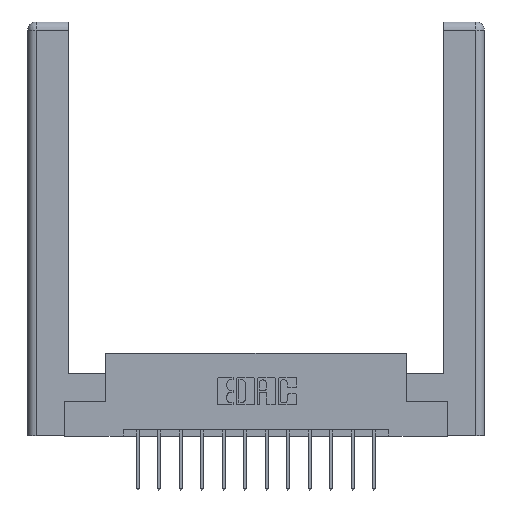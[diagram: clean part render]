
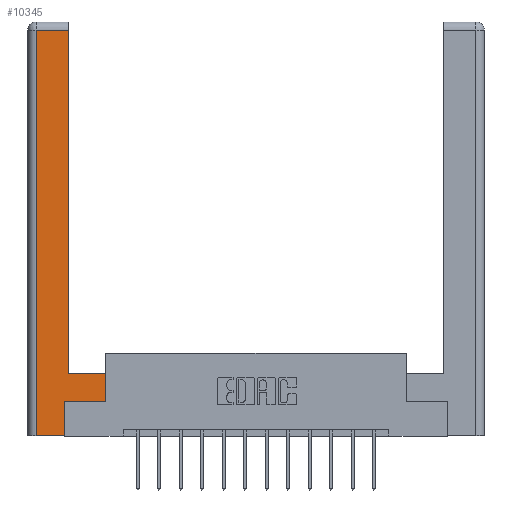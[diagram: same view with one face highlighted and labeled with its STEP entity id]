
A CAD part, top view. The second image highlights one B-rep face of the part: STEP entity #10345.
In plain terms, the highlighted planar face has unit normal (0, 0, 1).
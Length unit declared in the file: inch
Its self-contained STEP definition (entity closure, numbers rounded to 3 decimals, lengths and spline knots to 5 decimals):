
#161 = ORIENTED_EDGE ( 'NONE', *, *, #13510, .T. ) ;
#336 = DIRECTION ( 'NONE',  ( -1., 0., 0. ) ) ;
#454 = EDGE_CURVE ( 'NONE', #11372, #15323, #6470, .T. ) ;
#505 = CARTESIAN_POINT ( 'NONE',  ( 0.265, 0., 0. ) ) ;
#992 = CARTESIAN_POINT ( 'NONE',  ( 0.265, 0.245, 0. ) ) ;
#1476 = VERTEX_POINT ( 'NONE', #2406 ) ;
#1757 = VERTEX_POINT ( 'NONE', #505 ) ;
#1783 = LINE ( 'NONE', #3358, #5050 ) ;
#1943 = ORIENTED_EDGE ( 'NONE', *, *, #4255, .T. ) ;
#2093 = VECTOR ( 'NONE', #6991, 39.37008 ) ;
#2279 = VECTOR ( 'NONE', #3159, 39.37008 ) ;
#2306 = LINE ( 'NONE', #6156, #5923 ) ;
#2406 = CARTESIAN_POINT ( 'NONE',  ( 0.295, 0.45, 0. ) ) ;
#2756 = VERTEX_POINT ( 'NONE', #992 ) ;
#3066 = ORIENTED_EDGE ( 'NONE', *, *, #4370, .T. ) ;
#3159 = DIRECTION ( 'NONE',  ( 0., 1., 0. ) ) ;
#3294 = CARTESIAN_POINT ( 'NONE',  ( 0.565, 0.245, 0. ) ) ;
#3358 = CARTESIAN_POINT ( 'NONE',  ( 0.265, 0.245, 0. ) ) ;
#3514 = AXIS2_PLACEMENT_3D ( 'NONE', #7542, #14059, #6756 ) ;
#4255 = EDGE_CURVE ( 'NONE', #1476, #11372, #9552, .T. ) ;
#4336 = VERTEX_POINT ( 'NONE', #8377 ) ;
#4370 = EDGE_CURVE ( 'NONE', #15323, #4336, #6119, .T. ) ;
#4674 = DIRECTION ( 'NONE',  ( -1., 0., 0. ) ) ;
#5003 = VERTEX_POINT ( 'NONE', #10458 ) ;
#5050 = VECTOR ( 'NONE', #13098, 39.37008 ) ;
#5762 = FACE_OUTER_BOUND ( 'NONE', #10119, .T. ) ;
#5923 = VECTOR ( 'NONE', #14624, 39.37008 ) ;
#6119 = LINE ( 'NONE', #14278, #2093 ) ;
#6148 = PLANE ( 'NONE',  #3514 ) ;
#6156 = CARTESIAN_POINT ( 'NONE',  ( 0.265, 0., 0. ) ) ;
#6237 = LINE ( 'NONE', #3294, #15763 ) ;
#6454 = CARTESIAN_POINT ( 'NONE',  ( 0.295, 2.94, 0. ) ) ;
#6470 = LINE ( 'NONE', #15001, #13511 ) ;
#6756 = DIRECTION ( 'NONE',  ( -1., 0., 0. ) ) ;
#6791 = CARTESIAN_POINT ( 'NONE',  ( 0.295, 3., 0. ) ) ;
#6991 = DIRECTION ( 'NONE',  ( 0., -1., 0. ) ) ;
#7121 = LINE ( 'NONE', #10506, #12270 ) ;
#7542 = CARTESIAN_POINT ( 'NONE',  ( 0., 0., 0. ) ) ;
#7871 = ORIENTED_EDGE ( 'NONE', *, *, #9267, .T. ) ;
#8116 = EDGE_CURVE ( 'NONE', #1757, #2756, #1783, .T. ) ;
#8163 = DIRECTION ( 'NONE',  ( 1., 0., 0. ) ) ;
#8377 = CARTESIAN_POINT ( 'NONE',  ( 0.0615, 0., 0. ) ) ;
#9267 = EDGE_CURVE ( 'NONE', #12775, #5003, #7121, .T. ) ;
#9369 = ORIENTED_EDGE ( 'NONE', *, *, #8116, .T. ) ;
#9552 = LINE ( 'NONE', #6791, #2279 ) ;
#10119 = EDGE_LOOP ( 'NONE', ( #1943, #12083, #3066, #10430, #9369, #161, #7871, #10881 ) ) ;
#10345 = ADVANCED_FACE ( 'NONE', ( #5762 ), #6148, .F. ) ;
#10430 = ORIENTED_EDGE ( 'NONE', *, *, #14941, .T. ) ;
#10458 = CARTESIAN_POINT ( 'NONE',  ( 0.565, 0.45, 0. ) ) ;
#10506 = CARTESIAN_POINT ( 'NONE',  ( 0.565, 0.45, 0. ) ) ;
#10679 = CARTESIAN_POINT ( 'NONE',  ( 0.0615, 2.94, 0. ) ) ;
#10881 = ORIENTED_EDGE ( 'NONE', *, *, #13415, .T. ) ;
#11372 = VERTEX_POINT ( 'NONE', #6454 ) ;
#11906 = CARTESIAN_POINT ( 'NONE',  ( 0.565, 0.245, 0. ) ) ;
#11992 = CARTESIAN_POINT ( 'NONE',  ( 0.295, 0.45, 0. ) ) ;
#12083 = ORIENTED_EDGE ( 'NONE', *, *, #454, .T. ) ;
#12270 = VECTOR ( 'NONE', #15451, 39.37008 ) ;
#12341 = LINE ( 'NONE', #11992, #12710 ) ;
#12710 = VECTOR ( 'NONE', #4674, 39.37008 ) ;
#12775 = VERTEX_POINT ( 'NONE', #11906 ) ;
#13098 = DIRECTION ( 'NONE',  ( 0., 1., 0. ) ) ;
#13415 = EDGE_CURVE ( 'NONE', #5003, #1476, #12341, .T. ) ;
#13510 = EDGE_CURVE ( 'NONE', #2756, #12775, #6237, .T. ) ;
#13511 = VECTOR ( 'NONE', #336, 39.37008 ) ;
#14059 = DIRECTION ( 'NONE',  ( 0., 0., -1. ) ) ;
#14278 = CARTESIAN_POINT ( 'NONE',  ( 0.0615, 0., 0. ) ) ;
#14624 = DIRECTION ( 'NONE',  ( 1., 0., 0. ) ) ;
#14941 = EDGE_CURVE ( 'NONE', #4336, #1757, #2306, .T. ) ;
#15001 = CARTESIAN_POINT ( 'NONE',  ( 0.0615, 2.94, 0. ) ) ;
#15323 = VERTEX_POINT ( 'NONE', #10679 ) ;
#15451 = DIRECTION ( 'NONE',  ( 0., 1., 0. ) ) ;
#15763 = VECTOR ( 'NONE', #8163, 39.37008 ) ;
